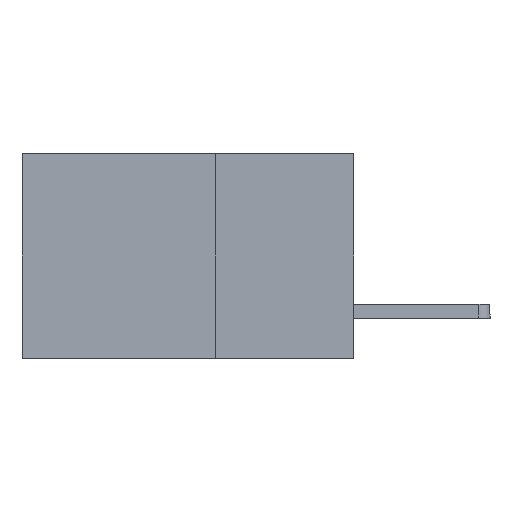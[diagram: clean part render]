
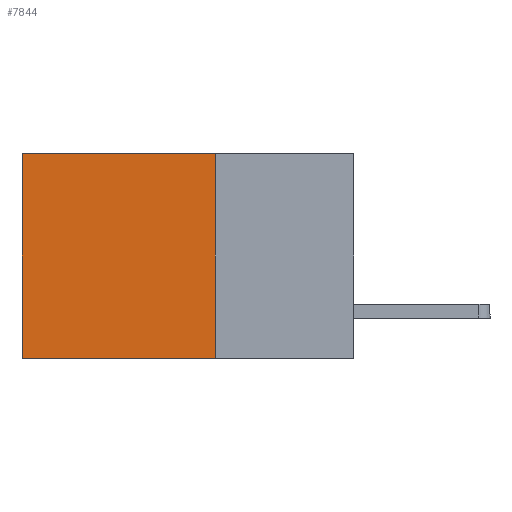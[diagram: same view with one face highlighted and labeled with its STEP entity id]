
A CAD part, left-side view. The second image highlights one B-rep face of the part: STEP entity #7844.
In plain terms, the highlighted planar face has unit normal (-1, 0, 0).
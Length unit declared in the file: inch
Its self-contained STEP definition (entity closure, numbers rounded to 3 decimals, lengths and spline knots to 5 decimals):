
#455 = VECTOR ( 'NONE', #10793, 39.37008 ) ;
#913 = ORIENTED_EDGE ( 'NONE', *, *, #11601, .T. ) ;
#1246 = VERTEX_POINT ( 'NONE', #7589 ) ;
#1772 = CARTESIAN_POINT ( 'NONE',  ( 0.2875, 0.25, 0. ) ) ;
#1960 = VECTOR ( 'NONE', #3841, 39.37008 ) ;
#1978 = CARTESIAN_POINT ( 'NONE',  ( 0.2875, 0.6, 0. ) ) ;
#2396 = EDGE_CURVE ( 'NONE', #3037, #5954, #7373, .T. ) ;
#3037 = VERTEX_POINT ( 'NONE', #1978 ) ;
#3315 = DIRECTION ( 'NONE',  ( 0., 1., 0. ) ) ;
#3324 = ORIENTED_EDGE ( 'NONE', *, *, #3394, .F. ) ;
#3394 = EDGE_CURVE ( 'NONE', #5689, #5954, #5849, .T. ) ;
#3841 = DIRECTION ( 'NONE',  ( 0., 1., 0. ) ) ;
#3937 = ORIENTED_EDGE ( 'NONE', *, *, #6560, .F. ) ;
#3945 = FACE_OUTER_BOUND ( 'NONE', #5855, .T. ) ;
#4582 = PLANE ( 'NONE',  #5367 ) ;
#4989 = VECTOR ( 'NONE', #5442, 39.37008 ) ;
#5367 = AXIS2_PLACEMENT_3D ( 'NONE', #1772, #10763, #5528 ) ;
#5442 = DIRECTION ( 'NONE',  ( 0., 0., -1. ) ) ;
#5528 = DIRECTION ( 'NONE',  ( 0., 0., -1. ) ) ;
#5553 = VECTOR ( 'NONE', #3315, 39.37008 ) ;
#5689 = VERTEX_POINT ( 'NONE', #7423 ) ;
#5737 = ORIENTED_EDGE ( 'NONE', *, *, #2396, .T. ) ;
#5740 = CARTESIAN_POINT ( 'NONE',  ( 0.2875, 0.6, 0. ) ) ;
#5849 = LINE ( 'NONE', #10499, #5553 ) ;
#5855 = EDGE_LOOP ( 'NONE', ( #5737, #3324, #3937, #913 ) ) ;
#5954 = VERTEX_POINT ( 'NONE', #10524 ) ;
#6560 = EDGE_CURVE ( 'NONE', #1246, #5689, #7829, .T. ) ;
#6606 = CARTESIAN_POINT ( 'NONE',  ( 0.2875, 0.25, 0. ) ) ;
#7142 = LINE ( 'NONE', #6606, #1960 ) ;
#7373 = LINE ( 'NONE', #5740, #4989 ) ;
#7423 = CARTESIAN_POINT ( 'NONE',  ( 0.2875, 0.25, -0.37 ) ) ;
#7589 = CARTESIAN_POINT ( 'NONE',  ( 0.2875, 0.25, 0. ) ) ;
#7829 = LINE ( 'NONE', #9931, #455 ) ;
#7844 = ADVANCED_FACE ( 'NONE', ( #3945 ), #4582, .F. ) ;
#9931 = CARTESIAN_POINT ( 'NONE',  ( 0.2875, 0.25, 0. ) ) ;
#10499 = CARTESIAN_POINT ( 'NONE',  ( 0.2875, 0.25, -0.37 ) ) ;
#10524 = CARTESIAN_POINT ( 'NONE',  ( 0.2875, 0.6, -0.37 ) ) ;
#10763 = DIRECTION ( 'NONE',  ( 1., 0., 0. ) ) ;
#10793 = DIRECTION ( 'NONE',  ( 0., 0., -1. ) ) ;
#11601 = EDGE_CURVE ( 'NONE', #1246, #3037, #7142, .T. ) ;
